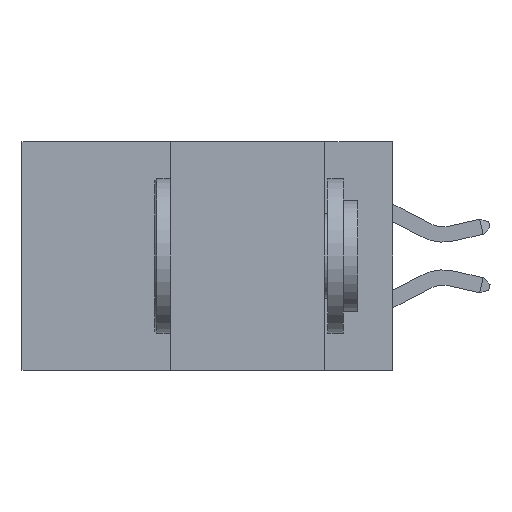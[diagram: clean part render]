
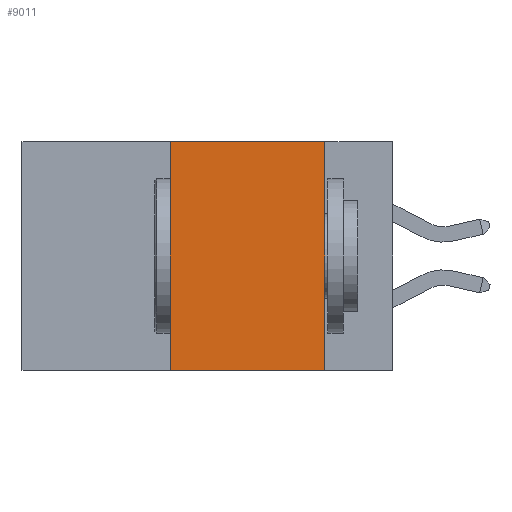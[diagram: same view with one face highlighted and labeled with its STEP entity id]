
A CAD part, left-side view. The second image highlights one B-rep face of the part: STEP entity #9011.
In plain terms, the highlighted planar face has unit normal (-1, 0, 0).
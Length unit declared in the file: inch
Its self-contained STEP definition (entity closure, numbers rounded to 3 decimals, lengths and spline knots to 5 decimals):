
#58 = CARTESIAN_POINT ( 'NONE',  ( 0., 0.11, 0. ) ) ;
#71 = VECTOR ( 'NONE', #2729, 39.37008 ) ;
#505 = DIRECTION ( 'NONE',  ( 0., 0., -1. ) ) ;
#515 = CARTESIAN_POINT ( 'NONE',  ( 0., 0.6, 0. ) ) ;
#1147 = DIRECTION ( 'NONE',  ( 0., 0., 1. ) ) ;
#1275 = LINE ( 'NONE', #8956, #4512 ) ;
#1306 = DIRECTION ( 'NONE',  ( 1., 0., 0. ) ) ;
#1671 = DIRECTION ( 'NONE',  ( 0., 0., -1. ) ) ;
#1799 = VECTOR ( 'NONE', #1147, 39.37008 ) ;
#2729 = DIRECTION ( 'NONE',  ( 0., -1., 0. ) ) ;
#2768 = EDGE_LOOP ( 'NONE', ( #3126, #6908, #4137, #5890 ) ) ;
#3126 = ORIENTED_EDGE ( 'NONE', *, *, #5742, .F. ) ;
#3279 = CARTESIAN_POINT ( 'NONE',  ( 0., 0.36, 0. ) ) ;
#4135 = VERTEX_POINT ( 'NONE', #58 ) ;
#4137 = ORIENTED_EDGE ( 'NONE', *, *, #4186, .F. ) ;
#4186 = EDGE_CURVE ( 'NONE', #7764, #8812, #7901, .T. ) ;
#4512 = VECTOR ( 'NONE', #4584, 39.37008 ) ;
#4584 = DIRECTION ( 'NONE',  ( 0., -1., 0. ) ) ;
#4864 = VERTEX_POINT ( 'NONE', #7385 ) ;
#5460 = EDGE_CURVE ( 'NONE', #7764, #4864, #1275, .T. ) ;
#5742 = EDGE_CURVE ( 'NONE', #4135, #4864, #8360, .T. ) ;
#5872 = FACE_OUTER_BOUND ( 'NONE', #2768, .T. ) ;
#5890 = ORIENTED_EDGE ( 'NONE', *, *, #5460, .T. ) ;
#6159 = LINE ( 'NONE', #515, #71 ) ;
#6165 = CARTESIAN_POINT ( 'NONE',  ( 0., 0.36, -0.37 ) ) ;
#6256 = CARTESIAN_POINT ( 'NONE',  ( 0., 0.11, 0. ) ) ;
#6810 = EDGE_CURVE ( 'NONE', #8812, #4135, #6159, .T. ) ;
#6908 = ORIENTED_EDGE ( 'NONE', *, *, #6810, .F. ) ;
#7175 = CARTESIAN_POINT ( 'NONE',  ( 0., 0.36, 0. ) ) ;
#7385 = CARTESIAN_POINT ( 'NONE',  ( 0., 0.11, -0.37 ) ) ;
#7764 = VERTEX_POINT ( 'NONE', #6165 ) ;
#7901 = LINE ( 'NONE', #7175, #1799 ) ;
#8360 = LINE ( 'NONE', #6256, #9675 ) ;
#8470 = AXIS2_PLACEMENT_3D ( 'NONE', #9017, #1306, #505 ) ;
#8812 = VERTEX_POINT ( 'NONE', #3279 ) ;
#8883 = PLANE ( 'NONE',  #8470 ) ;
#8956 = CARTESIAN_POINT ( 'NONE',  ( 0., 0.6, -0.37 ) ) ;
#9011 = ADVANCED_FACE ( 'NONE', ( #5872 ), #8883, .F. ) ;
#9017 = CARTESIAN_POINT ( 'NONE',  ( 0., 0.6, 0. ) ) ;
#9675 = VECTOR ( 'NONE', #1671, 39.37008 ) ;
